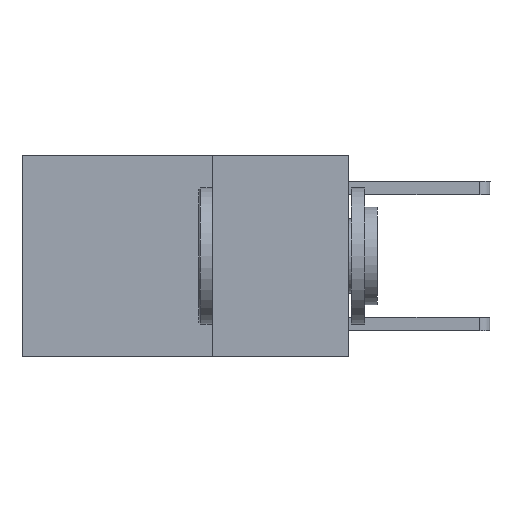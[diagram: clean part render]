
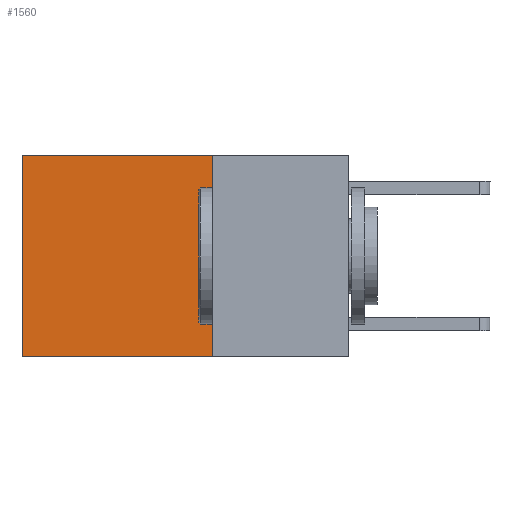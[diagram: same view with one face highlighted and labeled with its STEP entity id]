
A CAD part, left-side view. The second image highlights one B-rep face of the part: STEP entity #1560.
In plain terms, the highlighted planar face has unit normal (-1, 0, 0).
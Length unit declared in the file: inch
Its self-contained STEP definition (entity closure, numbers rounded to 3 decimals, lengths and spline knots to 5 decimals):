
#63 = VERTEX_POINT ( 'NONE', #2004 ) ;
#192 = CARTESIAN_POINT ( 'NONE',  ( 0.2625, 0.25, 0. ) ) ;
#363 = EDGE_CURVE ( 'NONE', #5169, #63, #1259, .T. ) ;
#548 = LINE ( 'NONE', #6416, #1026 ) ;
#631 = ORIENTED_EDGE ( 'NONE', *, *, #2280, .F. ) ;
#960 = LINE ( 'NONE', #2305, #4739 ) ;
#1026 = VECTOR ( 'NONE', #5602, 39.37008 ) ;
#1259 = LINE ( 'NONE', #4143, #6856 ) ;
#1368 = CARTESIAN_POINT ( 'NONE',  ( 0.2625, 0.25, 0. ) ) ;
#1560 = ADVANCED_FACE ( 'NONE', ( #5104 ), #3487, .F. ) ;
#1567 = DIRECTION ( 'NONE',  ( 0., 0., -1. ) ) ;
#1754 = EDGE_CURVE ( 'NONE', #63, #8937, #960, .T. ) ;
#1978 = CARTESIAN_POINT ( 'NONE',  ( 0.2625, 0.25, -0.37 ) ) ;
#2004 = CARTESIAN_POINT ( 'NONE',  ( 0.2625, 0.6, 0. ) ) ;
#2280 = EDGE_CURVE ( 'NONE', #7610, #8937, #548, .T. ) ;
#2305 = CARTESIAN_POINT ( 'NONE',  ( 0.2625, 0.6, 0. ) ) ;
#3487 = PLANE ( 'NONE',  #3696 ) ;
#3696 = AXIS2_PLACEMENT_3D ( 'NONE', #1368, #4295, #7360 ) ;
#3836 = DIRECTION ( 'NONE',  ( 0., 0., -1. ) ) ;
#4143 = CARTESIAN_POINT ( 'NONE',  ( 0.2625, 0.25, 0. ) ) ;
#4295 = DIRECTION ( 'NONE',  ( 1., 0., 0. ) ) ;
#4739 = VECTOR ( 'NONE', #3836, 39.37008 ) ;
#5104 = FACE_OUTER_BOUND ( 'NONE', #5352, .T. ) ;
#5169 = VERTEX_POINT ( 'NONE', #192 ) ;
#5352 = EDGE_LOOP ( 'NONE', ( #5509, #631, #6301, #7643 ) ) ;
#5509 = ORIENTED_EDGE ( 'NONE', *, *, #1754, .T. ) ;
#5515 = CARTESIAN_POINT ( 'NONE',  ( 0.2625, 0.6, -0.37 ) ) ;
#5602 = DIRECTION ( 'NONE',  ( 0., 1., 0. ) ) ;
#6301 = ORIENTED_EDGE ( 'NONE', *, *, #8689, .F. ) ;
#6416 = CARTESIAN_POINT ( 'NONE',  ( 0.2625, 0.25, -0.37 ) ) ;
#6856 = VECTOR ( 'NONE', #7119, 39.37008 ) ;
#7119 = DIRECTION ( 'NONE',  ( 0., 1., 0. ) ) ;
#7360 = DIRECTION ( 'NONE',  ( 0., 0., -1. ) ) ;
#7425 = VECTOR ( 'NONE', #1567, 39.37008 ) ;
#7610 = VERTEX_POINT ( 'NONE', #1978 ) ;
#7643 = ORIENTED_EDGE ( 'NONE', *, *, #363, .T. ) ;
#8064 = LINE ( 'NONE', #8960, #7425 ) ;
#8689 = EDGE_CURVE ( 'NONE', #5169, #7610, #8064, .T. ) ;
#8937 = VERTEX_POINT ( 'NONE', #5515 ) ;
#8960 = CARTESIAN_POINT ( 'NONE',  ( 0.2625, 0.25, 0. ) ) ;
